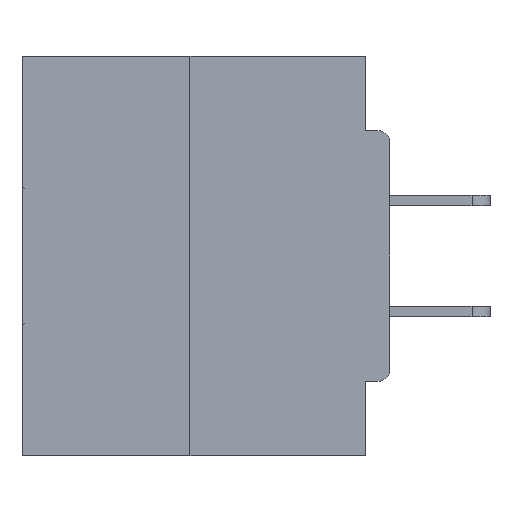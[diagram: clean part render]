
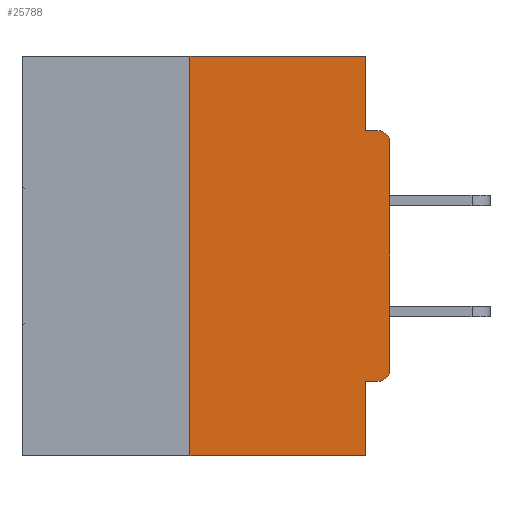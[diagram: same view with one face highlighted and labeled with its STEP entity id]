
A CAD part, left-side view. The second image highlights one B-rep face of the part: STEP entity #25788.
In plain terms, the highlighted planar face has unit normal (-1, 0, 0).
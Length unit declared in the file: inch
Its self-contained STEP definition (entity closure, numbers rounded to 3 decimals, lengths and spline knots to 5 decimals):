
#60 = CARTESIAN_POINT ( 'NONE',  ( 0., 0.46, 0. ) ) ;
#190 = ORIENTED_EDGE ( 'NONE', *, *, #39638, .F. ) ;
#1069 = CARTESIAN_POINT ( 'NONE',  ( 0., 0., -0.0935 ) ) ;
#1220 = EDGE_CURVE ( 'NONE', #1424, #26555, #30240, .T. ) ;
#1424 = VERTEX_POINT ( 'NONE', #35720 ) ;
#2986 = AXIS2_PLACEMENT_3D ( 'NONE', #32465, #13199, #38978 ) ;
#5010 = CARTESIAN_POINT ( 'NONE',  ( 0., 0.015, -0.0935 ) ) ;
#5920 = EDGE_CURVE ( 'NONE', #38570, #9143, #14724, .T. ) ;
#6503 = DIRECTION ( 'NONE',  ( 0., -1., 0. ) ) ;
#6803 = VERTEX_POINT ( 'NONE', #32202 ) ;
#7077 = CARTESIAN_POINT ( 'NONE',  ( 0., 0., -0.3915 ) ) ;
#7918 = CARTESIAN_POINT ( 'NONE',  ( 0., 0.015, -0.1085 ) ) ;
#8066 = DIRECTION ( 'NONE',  ( -1., 0., 0. ) ) ;
#8105 = ORIENTED_EDGE ( 'NONE', *, *, #35055, .F. ) ;
#8220 = ORIENTED_EDGE ( 'NONE', *, *, #9261, .T. ) ;
#8408 = DIRECTION ( 'NONE',  ( 0., 0., -1. ) ) ;
#8786 = LINE ( 'NONE', #60, #34967 ) ;
#9143 = VERTEX_POINT ( 'NONE', #7077 ) ;
#9261 = EDGE_CURVE ( 'NONE', #24116, #21153, #32782, .T. ) ;
#9673 = EDGE_CURVE ( 'NONE', #1424, #6803, #27776, .T. ) ;
#10058 = CARTESIAN_POINT ( 'NONE',  ( 0., 0., -0.4065 ) ) ;
#10121 = CARTESIAN_POINT ( 'NONE',  ( 0., 0., 0. ) ) ;
#10800 = VECTOR ( 'NONE', #20461, 39.37008 ) ;
#11392 = CARTESIAN_POINT ( 'NONE',  ( 0., 0.015, -0.3915 ) ) ;
#11429 = CARTESIAN_POINT ( 'NONE',  ( 0., 0.031, 0. ) ) ;
#11447 = DIRECTION ( 'NONE',  ( 0., 0., -1. ) ) ;
#13199 = DIRECTION ( 'NONE',  ( 1., 0., 0. ) ) ;
#13919 = AXIS2_PLACEMENT_3D ( 'NONE', #7918, #8066, #11447 ) ;
#14724 = CIRCLE ( 'NONE', #16816, 0.015 ) ;
#16162 = CARTESIAN_POINT ( 'NONE',  ( 0., 0.031, -0.0935 ) ) ;
#16816 = AXIS2_PLACEMENT_3D ( 'NONE', #11392, #34015, #40672 ) ;
#17856 = VERTEX_POINT ( 'NONE', #16162 ) ;
#18368 = VERTEX_POINT ( 'NONE', #37562 ) ;
#19074 = CARTESIAN_POINT ( 'NONE',  ( 0., 0.46, -0.5 ) ) ;
#19763 = DIRECTION ( 'NONE',  ( 0., 1., 0. ) ) ;
#19854 = ORIENTED_EDGE ( 'NONE', *, *, #39369, .F. ) ;
#20044 = EDGE_CURVE ( 'NONE', #38570, #18368, #25171, .T. ) ;
#20461 = DIRECTION ( 'NONE',  ( 0., -1., 0. ) ) ;
#20847 = VECTOR ( 'NONE', #38687, 39.37008 ) ;
#20983 = LINE ( 'NONE', #11429, #28519 ) ;
#21073 = CARTESIAN_POINT ( 'NONE',  ( 0., 0.031, -0.5 ) ) ;
#21153 = VERTEX_POINT ( 'NONE', #5010 ) ;
#21246 = VECTOR ( 'NONE', #39557, 39.37008 ) ;
#21497 = ORIENTED_EDGE ( 'NONE', *, *, #33545, .F. ) ;
#23357 = LINE ( 'NONE', #1069, #10800 ) ;
#23781 = CARTESIAN_POINT ( 'NONE',  ( 0., 0.015, -0.4065 ) ) ;
#24116 = VERTEX_POINT ( 'NONE', #32638 ) ;
#24632 = DIRECTION ( 'NONE',  ( 0., 0., -1. ) ) ;
#25171 = LINE ( 'NONE', #10058, #36791 ) ;
#25339 = ORIENTED_EDGE ( 'NONE', *, *, #1220, .T. ) ;
#25708 = DIRECTION ( 'NONE',  ( 0., -1., 0. ) ) ;
#25788 = ADVANCED_FACE ( 'NONE', ( #28619 ), #29230, .F. ) ;
#26555 = VERTEX_POINT ( 'NONE', #28881 ) ;
#27386 = LINE ( 'NONE', #10121, #20847 ) ;
#27776 = LINE ( 'NONE', #36292, #21246 ) ;
#28345 = LINE ( 'NONE', #21073, #38954 ) ;
#28433 = ORIENTED_EDGE ( 'NONE', *, *, #33440, .T. ) ;
#28519 = VECTOR ( 'NONE', #24632, 39.37008 ) ;
#28619 = FACE_OUTER_BOUND ( 'NONE', #31244, .T. ) ;
#28881 = CARTESIAN_POINT ( 'NONE',  ( 0., 0.031, -0.5 ) ) ;
#29230 = PLANE ( 'NONE',  #2986 ) ;
#29389 = ORIENTED_EDGE ( 'NONE', *, *, #5920, .T. ) ;
#30240 = LINE ( 'NONE', #19074, #37782 ) ;
#31024 = ORIENTED_EDGE ( 'NONE', *, *, #9673, .F. ) ;
#31244 = EDGE_LOOP ( 'NONE', ( #19854, #31024, #25339, #21497, #37021, #29389, #28433, #8220, #190, #8105 ) ) ;
#32202 = CARTESIAN_POINT ( 'NONE',  ( 0., 0.25, 0. ) ) ;
#32465 = CARTESIAN_POINT ( 'NONE',  ( 0., 0.46, 0. ) ) ;
#32638 = CARTESIAN_POINT ( 'NONE',  ( 0., 0., -0.1085 ) ) ;
#32782 = CIRCLE ( 'NONE', #13919, 0.015 ) ;
#33440 = EDGE_CURVE ( 'NONE', #9143, #24116, #27386, .T. ) ;
#33545 = EDGE_CURVE ( 'NONE', #18368, #26555, #28345, .T. ) ;
#34015 = DIRECTION ( 'NONE',  ( -1., 0., 0. ) ) ;
#34967 = VECTOR ( 'NONE', #6503, 39.37008 ) ;
#35055 = EDGE_CURVE ( 'NONE', #40495, #17856, #20983, .T. ) ;
#35433 = CARTESIAN_POINT ( 'NONE',  ( 0., 0.031, 0. ) ) ;
#35720 = CARTESIAN_POINT ( 'NONE',  ( 0., 0.25, -0.5 ) ) ;
#36292 = CARTESIAN_POINT ( 'NONE',  ( 0., 0.25, 0. ) ) ;
#36791 = VECTOR ( 'NONE', #19763, 39.37008 ) ;
#37021 = ORIENTED_EDGE ( 'NONE', *, *, #20044, .F. ) ;
#37562 = CARTESIAN_POINT ( 'NONE',  ( 0., 0.031, -0.4065 ) ) ;
#37782 = VECTOR ( 'NONE', #25708, 39.37008 ) ;
#38570 = VERTEX_POINT ( 'NONE', #23781 ) ;
#38687 = DIRECTION ( 'NONE',  ( 0., 0., 1. ) ) ;
#38954 = VECTOR ( 'NONE', #8408, 39.37008 ) ;
#38978 = DIRECTION ( 'NONE',  ( 0., 0., -1. ) ) ;
#39369 = EDGE_CURVE ( 'NONE', #6803, #40495, #8786, .T. ) ;
#39557 = DIRECTION ( 'NONE',  ( 0., 0., 1. ) ) ;
#39638 = EDGE_CURVE ( 'NONE', #17856, #21153, #23357, .T. ) ;
#40495 = VERTEX_POINT ( 'NONE', #35433 ) ;
#40672 = DIRECTION ( 'NONE',  ( 0., 0., -1. ) ) ;
